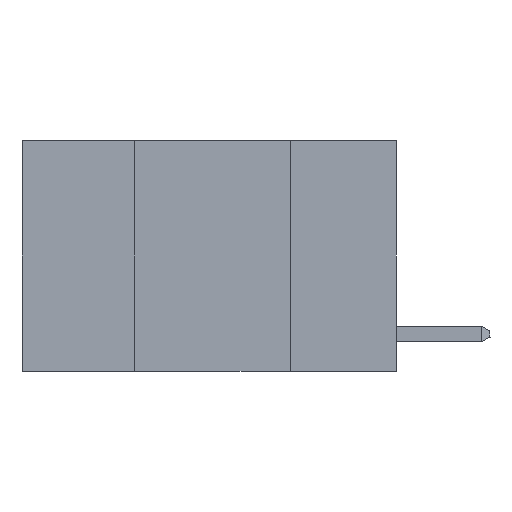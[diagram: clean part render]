
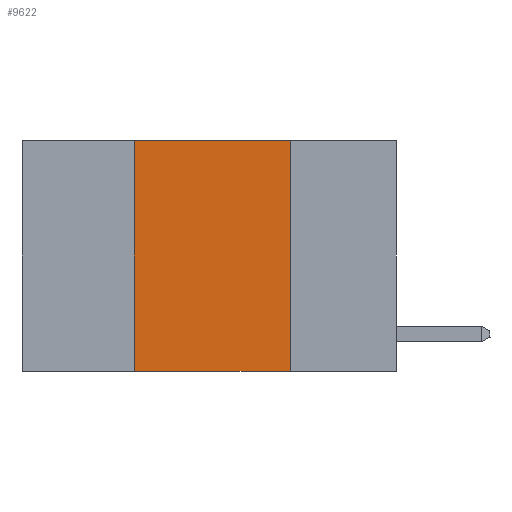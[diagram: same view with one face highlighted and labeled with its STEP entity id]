
A CAD part, left-side view. The second image highlights one B-rep face of the part: STEP entity #9622.
In plain terms, the highlighted planar face has unit normal (-1, 0, 0).
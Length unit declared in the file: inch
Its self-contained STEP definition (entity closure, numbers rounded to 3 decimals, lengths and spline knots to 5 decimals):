
#158 = PLANE ( 'NONE',  #2939 ) ;
#414 = FACE_OUTER_BOUND ( 'NONE', #4721, .T. ) ;
#728 = CARTESIAN_POINT ( 'NONE',  ( 0., 0.42, 0. ) ) ;
#879 = EDGE_CURVE ( 'NONE', #6238, #11343, #3501, .T. ) ;
#1398 = ORIENTED_EDGE ( 'NONE', *, *, #879, .F. ) ;
#1644 = EDGE_CURVE ( 'NONE', #2713, #3858, #10435, .T. ) ;
#1879 = ORIENTED_EDGE ( 'NONE', *, *, #4312, .F. ) ;
#2111 = ORIENTED_EDGE ( 'NONE', *, *, #1644, .F. ) ;
#2713 = VERTEX_POINT ( 'NONE', #3022 ) ;
#2718 = DIRECTION ( 'NONE',  ( 0., -1., 0. ) ) ;
#2939 = AXIS2_PLACEMENT_3D ( 'NONE', #3997, #3041, #3938 ) ;
#3022 = CARTESIAN_POINT ( 'NONE',  ( 0., 0.42, -0.37 ) ) ;
#3041 = DIRECTION ( 'NONE',  ( 1., 0., 0. ) ) ;
#3501 = LINE ( 'NONE', #7244, #11258 ) ;
#3693 = VECTOR ( 'NONE', #2718, 39.37008 ) ;
#3820 = DIRECTION ( 'NONE',  ( 0., 0., 1. ) ) ;
#3858 = VERTEX_POINT ( 'NONE', #728 ) ;
#3938 = DIRECTION ( 'NONE',  ( 0., 0., -1. ) ) ;
#3965 = CARTESIAN_POINT ( 'NONE',  ( 0., 0.17, 0. ) ) ;
#3997 = CARTESIAN_POINT ( 'NONE',  ( 0., 0.6, 0. ) ) ;
#4261 = ORIENTED_EDGE ( 'NONE', *, *, #5126, .T. ) ;
#4312 = EDGE_CURVE ( 'NONE', #3858, #6238, #9148, .T. ) ;
#4721 = EDGE_LOOP ( 'NONE', ( #1398, #1879, #2111, #4261 ) ) ;
#5126 = EDGE_CURVE ( 'NONE', #2713, #11343, #10047, .T. ) ;
#5659 = VECTOR ( 'NONE', #3820, 39.37008 ) ;
#6125 = VECTOR ( 'NONE', #10034, 39.37008 ) ;
#6238 = VERTEX_POINT ( 'NONE', #3965 ) ;
#7244 = CARTESIAN_POINT ( 'NONE',  ( 0., 0.17, 0. ) ) ;
#7313 = DIRECTION ( 'NONE',  ( 0., 0., -1. ) ) ;
#8325 = CARTESIAN_POINT ( 'NONE',  ( 0., 0.6, -0.37 ) ) ;
#8627 = CARTESIAN_POINT ( 'NONE',  ( 0., 0.42, 0. ) ) ;
#9148 = LINE ( 'NONE', #11910, #6125 ) ;
#9622 = ADVANCED_FACE ( 'NONE', ( #414 ), #158, .F. ) ;
#10034 = DIRECTION ( 'NONE',  ( 0., -1., 0. ) ) ;
#10047 = LINE ( 'NONE', #8325, #3693 ) ;
#10435 = LINE ( 'NONE', #8627, #5659 ) ;
#11064 = CARTESIAN_POINT ( 'NONE',  ( 0., 0.17, -0.37 ) ) ;
#11258 = VECTOR ( 'NONE', #7313, 39.37008 ) ;
#11343 = VERTEX_POINT ( 'NONE', #11064 ) ;
#11910 = CARTESIAN_POINT ( 'NONE',  ( 0., 0.6, 0. ) ) ;
